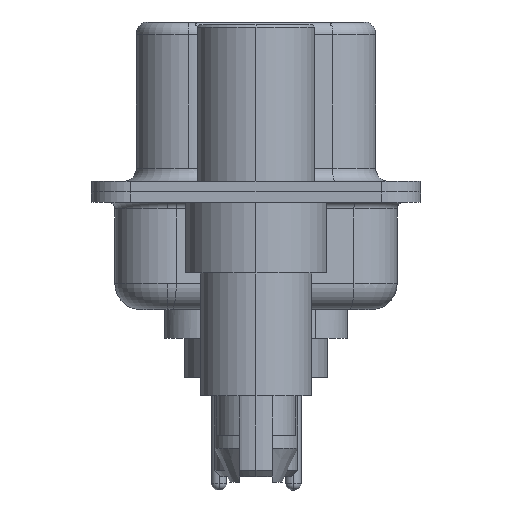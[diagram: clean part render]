
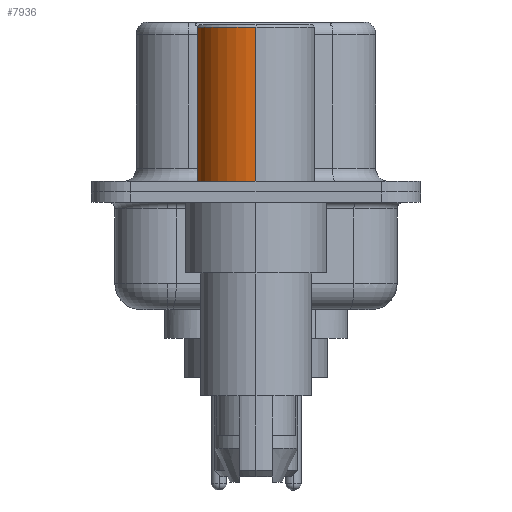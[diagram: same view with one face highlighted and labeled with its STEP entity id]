
A CAD part, left-side view. The second image highlights one B-rep face of the part: STEP entity #7936.
In plain terms, the highlighted cylindrical face has radius 2.25 mm (diameter 4.5 mm), a partial arc.
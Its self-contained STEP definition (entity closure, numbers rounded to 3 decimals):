
#242 = VERTEX_POINT ( 'NONE', #6954 ) ;
#758 = DIRECTION ( 'NONE',  ( 0., 0., 1. ) ) ;
#1194 = ORIENTED_EDGE ( 'NONE', *, *, #12641, .F. ) ;
#1562 = LINE ( 'NONE', #15062, #9054 ) ;
#1607 = DIRECTION ( 'NONE',  ( 0., 0., 1. ) ) ;
#3066 = LINE ( 'NONE', #4865, #14656 ) ;
#4865 = CARTESIAN_POINT ( 'NONE',  ( 2.25, 0., 0.581 ) ) ;
#4998 = CARTESIAN_POINT ( 'NONE',  ( 2.25, 0., 0.4 ) ) ;
#5169 = EDGE_CURVE ( 'NONE', #11987, #242, #18053, .T. ) ;
#5299 = CARTESIAN_POINT ( 'NONE',  ( 0., 0., 0.581 ) ) ;
#5730 = AXIS2_PLACEMENT_3D ( 'NONE', #5299, #758, #9748 ) ;
#6954 = CARTESIAN_POINT ( 'NONE',  ( -2.25, 0., 0.4 ) ) ;
#7495 = DIRECTION ( 'NONE',  ( 0., 0., 1. ) ) ;
#7715 = EDGE_CURVE ( 'NONE', #11987, #9203, #3066, .T. ) ;
#7719 = AXIS2_PLACEMENT_3D ( 'NONE', #14382, #9281, #7769 ) ;
#7769 = DIRECTION ( 'NONE',  ( 1., 0., 0. ) ) ;
#7936 = ADVANCED_FACE ( 'NONE', ( #12296 ), #15853, .T. ) ;
#8192 = CARTESIAN_POINT ( 'NONE',  ( 2.25, 0., 6.3 ) ) ;
#9054 = VECTOR ( 'NONE', #7495, 1000. ) ;
#9203 = VERTEX_POINT ( 'NONE', #8192 ) ;
#9281 = DIRECTION ( 'NONE',  ( 0., 0., 1. ) ) ;
#9748 = DIRECTION ( 'NONE',  ( 1., 0., 0. ) ) ;
#10099 = EDGE_LOOP ( 'NONE', ( #11626, #15228, #1194, #15936 ) ) ;
#10136 = EDGE_CURVE ( 'NONE', #242, #10554, #1562, .T. ) ;
#10554 = VERTEX_POINT ( 'NONE', #11896 ) ;
#10615 = CARTESIAN_POINT ( 'NONE',  ( 0., 0., 6.3 ) ) ;
#11626 = ORIENTED_EDGE ( 'NONE', *, *, #5169, .T. ) ;
#11896 = CARTESIAN_POINT ( 'NONE',  ( -2.25, 0., 6.3 ) ) ;
#11987 = VERTEX_POINT ( 'NONE', #4998 ) ;
#12182 = DIRECTION ( 'NONE',  ( 1., 0., 0. ) ) ;
#12296 = FACE_OUTER_BOUND ( 'NONE', #10099, .T. ) ;
#12641 = EDGE_CURVE ( 'NONE', #9203, #10554, #15183, .T. ) ;
#14382 = CARTESIAN_POINT ( 'NONE',  ( 0., 0., 0.4 ) ) ;
#14656 = VECTOR ( 'NONE', #18424, 1000. ) ;
#15062 = CARTESIAN_POINT ( 'NONE',  ( -2.25, 0., 0.581 ) ) ;
#15176 = AXIS2_PLACEMENT_3D ( 'NONE', #10615, #1607, #12182 ) ;
#15183 = CIRCLE ( 'NONE', #15176, 2.25 ) ;
#15228 = ORIENTED_EDGE ( 'NONE', *, *, #10136, .T. ) ;
#15853 = CYLINDRICAL_SURFACE ( 'NONE', #5730, 2.25 ) ;
#15936 = ORIENTED_EDGE ( 'NONE', *, *, #7715, .F. ) ;
#18053 = CIRCLE ( 'NONE', #7719, 2.25 ) ;
#18424 = DIRECTION ( 'NONE',  ( 0., 0., 1. ) ) ;
